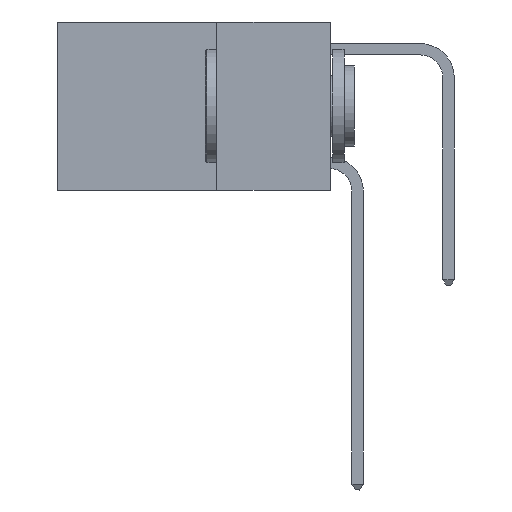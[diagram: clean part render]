
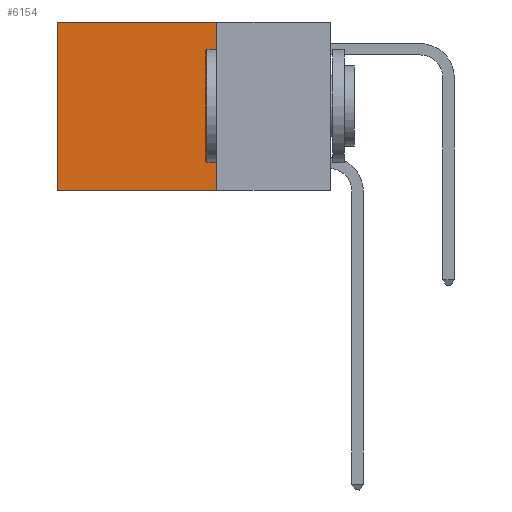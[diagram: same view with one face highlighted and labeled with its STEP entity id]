
A CAD part, left-side view. The second image highlights one B-rep face of the part: STEP entity #6154.
In plain terms, the highlighted planar face has unit normal (-1, 0, 0).
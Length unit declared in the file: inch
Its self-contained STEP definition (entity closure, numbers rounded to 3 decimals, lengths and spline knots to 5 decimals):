
#242 = VECTOR ( 'NONE', #1624, 39.37008 ) ;
#347 = EDGE_LOOP ( 'NONE', ( #16870, #16730, #10650, #10373 ) ) ;
#1364 = VECTOR ( 'NONE', #6417, 39.37008 ) ;
#1624 = DIRECTION ( 'NONE',  ( 0., 0., -1. ) ) ;
#2774 = VERTEX_POINT ( 'NONE', #17300 ) ;
#3074 = PLANE ( 'NONE',  #11185 ) ;
#4735 = EDGE_CURVE ( 'NONE', #2774, #10041, #12771, .T. ) ;
#5104 = LINE ( 'NONE', #15723, #1364 ) ;
#6154 = ADVANCED_FACE ( 'NONE', ( #15095 ), #3074, .F. ) ;
#6251 = CARTESIAN_POINT ( 'NONE',  ( 0.2625, 0.25, 0. ) ) ;
#6417 = DIRECTION ( 'NONE',  ( 0., 1., 0. ) ) ;
#6549 = VERTEX_POINT ( 'NONE', #7188 ) ;
#7188 = CARTESIAN_POINT ( 'NONE',  ( 0.2625, 0.25, -0.37 ) ) ;
#7815 = DIRECTION ( 'NONE',  ( 0., 0., -1. ) ) ;
#7819 = CARTESIAN_POINT ( 'NONE',  ( 0.2625, 0.25, 0. ) ) ;
#7907 = CARTESIAN_POINT ( 'NONE',  ( 0.2625, 0.6, 0. ) ) ;
#9432 = DIRECTION ( 'NONE',  ( 0., 0., -1. ) ) ;
#9605 = EDGE_CURVE ( 'NONE', #15842, #2774, #11785, .T. ) ;
#10041 = VERTEX_POINT ( 'NONE', #18132 ) ;
#10373 = ORIENTED_EDGE ( 'NONE', *, *, #9605, .T. ) ;
#10650 = ORIENTED_EDGE ( 'NONE', *, *, #10911, .F. ) ;
#10911 = EDGE_CURVE ( 'NONE', #15842, #6549, #13209, .T. ) ;
#11185 = AXIS2_PLACEMENT_3D ( 'NONE', #6251, #17074, #7815 ) ;
#11785 = LINE ( 'NONE', #15592, #15906 ) ;
#12771 = LINE ( 'NONE', #7907, #242 ) ;
#13209 = LINE ( 'NONE', #18611, #16810 ) ;
#13986 = DIRECTION ( 'NONE',  ( 0., 1., 0. ) ) ;
#14768 = EDGE_CURVE ( 'NONE', #6549, #10041, #5104, .T. ) ;
#15095 = FACE_OUTER_BOUND ( 'NONE', #347, .T. ) ;
#15592 = CARTESIAN_POINT ( 'NONE',  ( 0.2625, 0.25, 0. ) ) ;
#15723 = CARTESIAN_POINT ( 'NONE',  ( 0.2625, 0.25, -0.37 ) ) ;
#15842 = VERTEX_POINT ( 'NONE', #7819 ) ;
#15906 = VECTOR ( 'NONE', #13986, 39.37008 ) ;
#16730 = ORIENTED_EDGE ( 'NONE', *, *, #14768, .F. ) ;
#16810 = VECTOR ( 'NONE', #9432, 39.37008 ) ;
#16870 = ORIENTED_EDGE ( 'NONE', *, *, #4735, .T. ) ;
#17074 = DIRECTION ( 'NONE',  ( 1., 0., 0. ) ) ;
#17300 = CARTESIAN_POINT ( 'NONE',  ( 0.2625, 0.6, 0. ) ) ;
#18132 = CARTESIAN_POINT ( 'NONE',  ( 0.2625, 0.6, -0.37 ) ) ;
#18611 = CARTESIAN_POINT ( 'NONE',  ( 0.2625, 0.25, 0. ) ) ;
